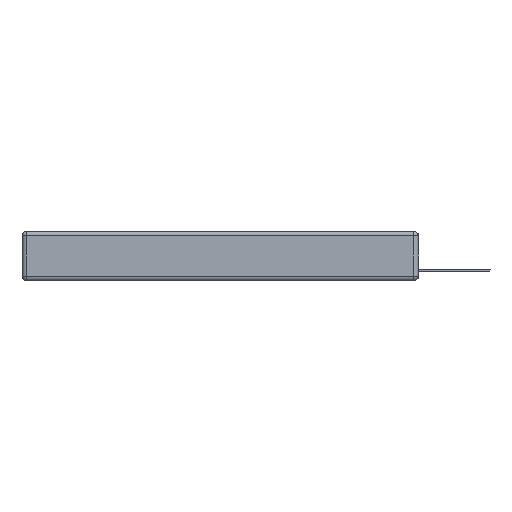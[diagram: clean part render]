
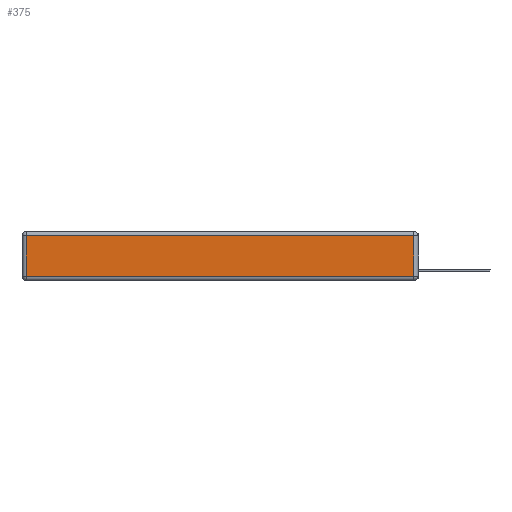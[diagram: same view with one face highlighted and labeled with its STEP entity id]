
A CAD part, left-side view. The second image highlights one B-rep face of the part: STEP entity #375.
In plain terms, the highlighted planar face has unit normal (-1, 0, 0).
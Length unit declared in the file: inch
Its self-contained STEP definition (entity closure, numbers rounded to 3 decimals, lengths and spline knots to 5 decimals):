
#375 = ADVANCED_FACE ( 'NONE', ( #23527 ), #5324, .T. ) ;
#1370 = EDGE_CURVE ( 'NONE', #18088, #23439, #3537, .T. ) ;
#1699 = CARTESIAN_POINT ( 'NONE',  ( 0., 0., -0.313 ) ) ;
#1980 = LINE ( 'NONE', #15953, #22746 ) ;
#3169 = ORIENTED_EDGE ( 'NONE', *, *, #1370, .T. ) ;
#3395 = CARTESIAN_POINT ( 'NONE',  ( 0., 2.72, -0.313 ) ) ;
#3537 = LINE ( 'NONE', #23733, #4643 ) ;
#4643 = VECTOR ( 'NONE', #21747, 39.37008 ) ;
#5159 = ORIENTED_EDGE ( 'NONE', *, *, #19184, .T. ) ;
#5324 = PLANE ( 'NONE',  #25678 ) ;
#5860 = EDGE_LOOP ( 'NONE', ( #24244, #15299, #3169, #5159 ) ) ;
#5960 = DIRECTION ( 'NONE',  ( 0., -1., 0. ) ) ;
#6325 = CARTESIAN_POINT ( 'NONE',  ( 0., 2.72, -0.03 ) ) ;
#6615 = CARTESIAN_POINT ( 'NONE',  ( 0., 0.03, -0.03 ) ) ;
#6948 = CARTESIAN_POINT ( 'NONE',  ( 0., 2.72, -0.343 ) ) ;
#9183 = CARTESIAN_POINT ( 'NONE',  ( 0., 0., -0.343 ) ) ;
#10939 = VERTEX_POINT ( 'NONE', #3395 ) ;
#13328 = LINE ( 'NONE', #6948, #15776 ) ;
#13672 = EDGE_CURVE ( 'NONE', #10939, #18644, #15936, .T. ) ;
#14099 = DIRECTION ( 'NONE',  ( 0., 0., 1. ) ) ;
#15067 = DIRECTION ( 'NONE',  ( 0., 0., -1. ) ) ;
#15299 = ORIENTED_EDGE ( 'NONE', *, *, #25374, .T. ) ;
#15776 = VECTOR ( 'NONE', #15067, 39.37008 ) ;
#15828 = DIRECTION ( 'NONE',  ( 0., 0., 1. ) ) ;
#15936 = LINE ( 'NONE', #1699, #20188 ) ;
#15953 = CARTESIAN_POINT ( 'NONE',  ( 0., 0.03, -0.343 ) ) ;
#16569 = CARTESIAN_POINT ( 'NONE',  ( 0., 0.03, -0.313 ) ) ;
#18088 = VERTEX_POINT ( 'NONE', #6615 ) ;
#18644 = VERTEX_POINT ( 'NONE', #16569 ) ;
#19184 = EDGE_CURVE ( 'NONE', #23439, #10939, #13328, .T. ) ;
#20188 = VECTOR ( 'NONE', #5960, 39.37008 ) ;
#21747 = DIRECTION ( 'NONE',  ( 0., 1., 0. ) ) ;
#22746 = VECTOR ( 'NONE', #14099, 39.37008 ) ;
#23439 = VERTEX_POINT ( 'NONE', #6325 ) ;
#23527 = FACE_OUTER_BOUND ( 'NONE', #5860, .T. ) ;
#23733 = CARTESIAN_POINT ( 'NONE',  ( 0., 2.75, -0.03 ) ) ;
#24244 = ORIENTED_EDGE ( 'NONE', *, *, #13672, .T. ) ;
#24314 = DIRECTION ( 'NONE',  ( -1., 0., 0. ) ) ;
#25374 = EDGE_CURVE ( 'NONE', #18644, #18088, #1980, .T. ) ;
#25678 = AXIS2_PLACEMENT_3D ( 'NONE', #9183, #24314, #15828 ) ;
